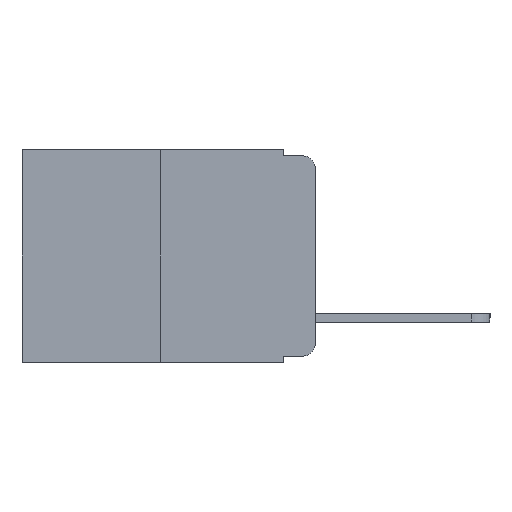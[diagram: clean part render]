
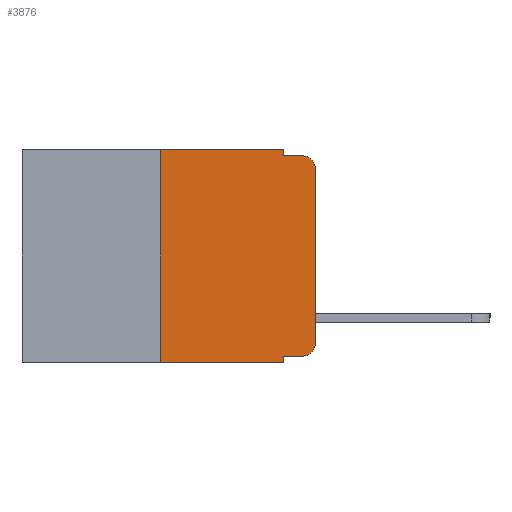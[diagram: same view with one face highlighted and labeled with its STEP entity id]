
A CAD part, left-side view. The second image highlights one B-rep face of the part: STEP entity #3876.
In plain terms, the highlighted planar face has unit normal (-1, 0, 0).
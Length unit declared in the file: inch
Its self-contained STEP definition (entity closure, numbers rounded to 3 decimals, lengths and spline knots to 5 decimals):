
#530 = LINE ( 'NONE', #5567, #17641 ) ;
#1153 = DIRECTION ( 'NONE',  ( 0., -1., 0. ) ) ;
#1159 = EDGE_CURVE ( 'NONE', #12731, #8257, #17762, .T. ) ;
#1178 = DIRECTION ( 'NONE',  ( 0., 0., -1. ) ) ;
#1666 = EDGE_CURVE ( 'NONE', #9956, #19249, #9150, .T. ) ;
#1695 = EDGE_CURVE ( 'NONE', #19249, #5350, #12815, .T. ) ;
#1701 = EDGE_CURVE ( 'NONE', #2002, #5350, #20406, .T. ) ;
#1781 = EDGE_CURVE ( 'NONE', #20860, #2002, #7636, .T. ) ;
#1883 = EDGE_CURVE ( 'NONE', #12731, #18690, #530, .T. ) ;
#1886 = EDGE_CURVE ( 'NONE', #14534, #8257, #4931, .T. ) ;
#1980 = EDGE_CURVE ( 'NONE', #14534, #4521, #20145, .T. ) ;
#2002 = VERTEX_POINT ( 'NONE', #7257 ) ;
#2011 = EDGE_CURVE ( 'NONE', #4521, #9956, #19701, .T. ) ;
#2292 = ORIENTED_EDGE ( 'NONE', *, *, #1695, .T. ) ;
#2469 = CARTESIAN_POINT ( 'NONE',  ( 0., 0.473, -0.343 ) ) ;
#2680 = DIRECTION ( 'NONE',  ( 0., -1., 0. ) ) ;
#2753 = EDGE_CURVE ( 'NONE', #18690, #20860, #5411, .T. ) ;
#3125 = AXIS2_PLACEMENT_3D ( 'NONE', #7945, #19191, #12534 ) ;
#3281 = CARTESIAN_POINT ( 'NONE',  ( 0., 0.02, -0.01 ) ) ;
#3495 = ORIENTED_EDGE ( 'NONE', *, *, #2753, .F. ) ;
#3876 = ADVANCED_FACE ( 'NONE', ( #20286 ), #18762, .F. ) ;
#4062 = ORIENTED_EDGE ( 'NONE', *, *, #1883, .F. ) ;
#4308 = VECTOR ( 'NONE', #11970, 39.37008 ) ;
#4521 = VERTEX_POINT ( 'NONE', #16982 ) ;
#4931 = LINE ( 'NONE', #17565, #21063 ) ;
#5350 = VERTEX_POINT ( 'NONE', #3281 ) ;
#5411 = LINE ( 'NONE', #16048, #4308 ) ;
#5567 = CARTESIAN_POINT ( 'NONE',  ( 0., 0.25, 0. ) ) ;
#6367 = DIRECTION ( 'NONE',  ( 0., 0., -1. ) ) ;
#6822 = ORIENTED_EDGE ( 'NONE', *, *, #2011, .T. ) ;
#7257 = CARTESIAN_POINT ( 'NONE',  ( 0., 0.051, -0.01 ) ) ;
#7636 = LINE ( 'NONE', #17434, #8159 ) ;
#7945 = CARTESIAN_POINT ( 'NONE',  ( 0., 0.02, -0.03 ) ) ;
#8159 = VECTOR ( 'NONE', #1178, 39.37008 ) ;
#8257 = VERTEX_POINT ( 'NONE', #19527 ) ;
#8263 = DIRECTION ( 'NONE',  ( 0., 0., -1. ) ) ;
#9062 = DIRECTION ( 'NONE',  ( 0., -1., 0. ) ) ;
#9150 = LINE ( 'NONE', #19819, #16906 ) ;
#9358 = DIRECTION ( 'NONE',  ( 1., 0., 0. ) ) ;
#9770 = CARTESIAN_POINT ( 'NONE',  ( 0., 0.051, 0. ) ) ;
#9956 = VERTEX_POINT ( 'NONE', #13396 ) ;
#10138 = ORIENTED_EDGE ( 'NONE', *, *, #1980, .T. ) ;
#10543 = AXIS2_PLACEMENT_3D ( 'NONE', #13759, #9358, #6367 ) ;
#10673 = EDGE_LOOP ( 'NONE', ( #19036, #2292, #11797, #19891, #3495, #4062, #12776, #17854, #10138, #6822 ) ) ;
#10691 = CARTESIAN_POINT ( 'NONE',  ( 0., 0.25, -0.343 ) ) ;
#10878 = AXIS2_PLACEMENT_3D ( 'NONE', #16530, #19673, #19504 ) ;
#11797 = ORIENTED_EDGE ( 'NONE', *, *, #1701, .F. ) ;
#11970 = DIRECTION ( 'NONE',  ( 0., -1., 0. ) ) ;
#12534 = DIRECTION ( 'NONE',  ( 0., 0., -1. ) ) ;
#12731 = VERTEX_POINT ( 'NONE', #10691 ) ;
#12776 = ORIENTED_EDGE ( 'NONE', *, *, #1159, .T. ) ;
#12815 = CIRCLE ( 'NONE', #3125, 0.02 ) ;
#13010 = CARTESIAN_POINT ( 'NONE',  ( 0., 0., -0.03 ) ) ;
#13396 = CARTESIAN_POINT ( 'NONE',  ( 0., 0., -0.313 ) ) ;
#13642 = VECTOR ( 'NONE', #2680, 39.37008 ) ;
#13759 = CARTESIAN_POINT ( 'NONE',  ( 0., 0.473, 0. ) ) ;
#14534 = VERTEX_POINT ( 'NONE', #14719 ) ;
#14719 = CARTESIAN_POINT ( 'NONE',  ( 0., 0.051, -0.333 ) ) ;
#15680 = VECTOR ( 'NONE', #1153, 39.37008 ) ;
#16048 = CARTESIAN_POINT ( 'NONE',  ( 0., 0.473, 0. ) ) ;
#16371 = DIRECTION ( 'NONE',  ( 0., 0., 1. ) ) ;
#16435 = VECTOR ( 'NONE', #9062, 39.37008 ) ;
#16530 = CARTESIAN_POINT ( 'NONE',  ( 0., 0.02, -0.313 ) ) ;
#16906 = VECTOR ( 'NONE', #18952, 39.37008 ) ;
#16982 = CARTESIAN_POINT ( 'NONE',  ( 0., 0.02, -0.333 ) ) ;
#17434 = CARTESIAN_POINT ( 'NONE',  ( 0., 0.051, 0. ) ) ;
#17565 = CARTESIAN_POINT ( 'NONE',  ( 0., 0.051, 0. ) ) ;
#17641 = VECTOR ( 'NONE', #16371, 39.37008 ) ;
#17762 = LINE ( 'NONE', #2469, #13642 ) ;
#17854 = ORIENTED_EDGE ( 'NONE', *, *, #1886, .F. ) ;
#18478 = CARTESIAN_POINT ( 'NONE',  ( 0., 0.051, -0.01 ) ) ;
#18690 = VERTEX_POINT ( 'NONE', #20632 ) ;
#18762 = PLANE ( 'NONE',  #10543 ) ;
#18952 = DIRECTION ( 'NONE',  ( 0., 0., 1. ) ) ;
#19036 = ORIENTED_EDGE ( 'NONE', *, *, #1666, .T. ) ;
#19191 = DIRECTION ( 'NONE',  ( -1., 0., 0. ) ) ;
#19249 = VERTEX_POINT ( 'NONE', #13010 ) ;
#19504 = DIRECTION ( 'NONE',  ( 0., 0., -1. ) ) ;
#19527 = CARTESIAN_POINT ( 'NONE',  ( 0., 0.051, -0.343 ) ) ;
#19673 = DIRECTION ( 'NONE',  ( -1., 0., 0. ) ) ;
#19701 = CIRCLE ( 'NONE', #10878, 0.02 ) ;
#19819 = CARTESIAN_POINT ( 'NONE',  ( 0., 0., 0. ) ) ;
#19891 = ORIENTED_EDGE ( 'NONE', *, *, #1781, .F. ) ;
#20145 = LINE ( 'NONE', #20396, #15680 ) ;
#20286 = FACE_OUTER_BOUND ( 'NONE', #10673, .T. ) ;
#20396 = CARTESIAN_POINT ( 'NONE',  ( 0., 0.051, -0.333 ) ) ;
#20406 = LINE ( 'NONE', #18478, #16435 ) ;
#20632 = CARTESIAN_POINT ( 'NONE',  ( 0., 0.25, 0. ) ) ;
#20860 = VERTEX_POINT ( 'NONE', #9770 ) ;
#21063 = VECTOR ( 'NONE', #8263, 39.37008 ) ;
